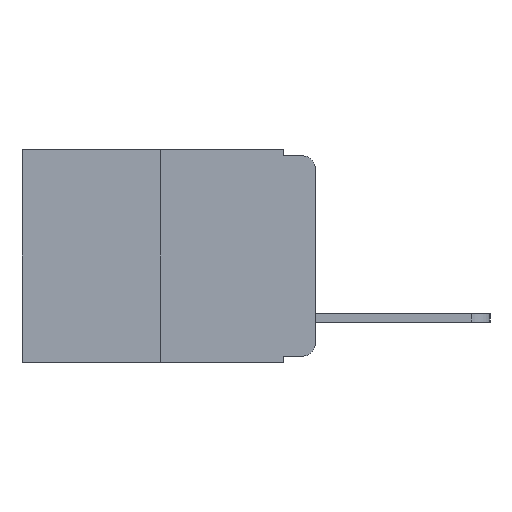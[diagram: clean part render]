
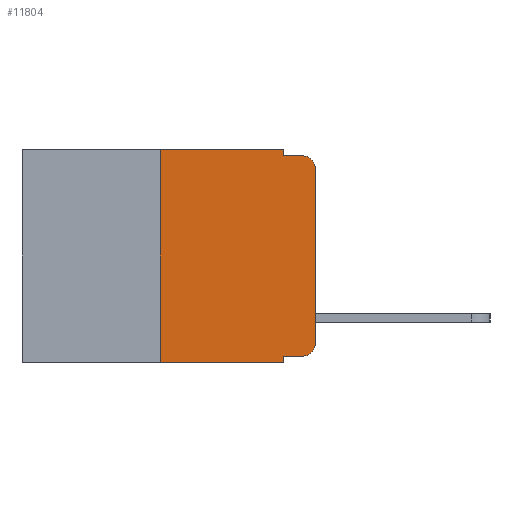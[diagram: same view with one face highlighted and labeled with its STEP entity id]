
A CAD part, left-side view. The second image highlights one B-rep face of the part: STEP entity #11804.
In plain terms, the highlighted planar face has unit normal (-1, 0, 0).
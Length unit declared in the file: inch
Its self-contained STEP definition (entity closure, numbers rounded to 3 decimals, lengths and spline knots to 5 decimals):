
#32 = CARTESIAN_POINT ( 'NONE',  ( 0., 0.051, -0.343 ) ) ;
#42 = DIRECTION ( 'NONE',  ( 0., -1., 0. ) ) ;
#110 = ORIENTED_EDGE ( 'NONE', *, *, #9940, .F. ) ;
#176 = CARTESIAN_POINT ( 'NONE',  ( 0., 0.473, -0.343 ) ) ;
#435 = DIRECTION ( 'NONE',  ( 0., -1., 0. ) ) ;
#461 = ORIENTED_EDGE ( 'NONE', *, *, #7917, .F. ) ;
#482 = CIRCLE ( 'NONE', #11625, 0.02 ) ;
#534 = VERTEX_POINT ( 'NONE', #5466 ) ;
#647 = ORIENTED_EDGE ( 'NONE', *, *, #4468, .T. ) ;
#747 = DIRECTION ( 'NONE',  ( 0., 0., -1. ) ) ;
#757 = DIRECTION ( 'NONE',  ( -1., 0., 0. ) ) ;
#991 = CARTESIAN_POINT ( 'NONE',  ( 0., 0.02, -0.313 ) ) ;
#1329 = EDGE_CURVE ( 'NONE', #7697, #7129, #11674, .T. ) ;
#1594 = LINE ( 'NONE', #12855, #9367 ) ;
#1974 = DIRECTION ( 'NONE',  ( 1., 0., 0. ) ) ;
#2759 = AXIS2_PLACEMENT_3D ( 'NONE', #12296, #1974, #9182 ) ;
#2839 = EDGE_CURVE ( 'NONE', #534, #7697, #7944, .T. ) ;
#3065 = ORIENTED_EDGE ( 'NONE', *, *, #1329, .T. ) ;
#3116 = DIRECTION ( 'NONE',  ( 0., -1., 0. ) ) ;
#3269 = DIRECTION ( 'NONE',  ( 0., 0., -1. ) ) ;
#3598 = LINE ( 'NONE', #3801, #8440 ) ;
#3801 = CARTESIAN_POINT ( 'NONE',  ( 0., 0.051, 0. ) ) ;
#3832 = LINE ( 'NONE', #6794, #9260 ) ;
#3987 = CARTESIAN_POINT ( 'NONE',  ( 0., 0.473, 0. ) ) ;
#4036 = ORIENTED_EDGE ( 'NONE', *, *, #6820, .F. ) ;
#4347 = ORIENTED_EDGE ( 'NONE', *, *, #5886, .F. ) ;
#4373 = DIRECTION ( 'NONE',  ( 0., -1., 0. ) ) ;
#4468 = EDGE_CURVE ( 'NONE', #10288, #534, #482, .T. ) ;
#5181 = EDGE_CURVE ( 'NONE', #6390, #10288, #1594, .T. ) ;
#5359 = VERTEX_POINT ( 'NONE', #7975 ) ;
#5466 = CARTESIAN_POINT ( 'NONE',  ( 0., 0., -0.313 ) ) ;
#5480 = CARTESIAN_POINT ( 'NONE',  ( 0., 0.02, -0.01 ) ) ;
#5528 = DIRECTION ( 'NONE',  ( 0., 0., -1. ) ) ;
#5850 = FACE_OUTER_BOUND ( 'NONE', #8494, .T. ) ;
#5886 = EDGE_CURVE ( 'NONE', #6390, #7399, #3598, .T. ) ;
#6109 = CARTESIAN_POINT ( 'NONE',  ( 0., 0.051, -0.333 ) ) ;
#6182 = VECTOR ( 'NONE', #42, 39.37008 ) ;
#6390 = VERTEX_POINT ( 'NONE', #6109 ) ;
#6794 = CARTESIAN_POINT ( 'NONE',  ( 0., 0.051, -0.01 ) ) ;
#6820 = EDGE_CURVE ( 'NONE', #7747, #5359, #8273, .T. ) ;
#6952 = CARTESIAN_POINT ( 'NONE',  ( 0., 0.02, -0.333 ) ) ;
#7085 = ORIENTED_EDGE ( 'NONE', *, *, #5181, .T. ) ;
#7104 = PLANE ( 'NONE',  #2759 ) ;
#7129 = VERTEX_POINT ( 'NONE', #5480 ) ;
#7214 = EDGE_CURVE ( 'NONE', #12556, #7747, #9479, .T. ) ;
#7241 = CARTESIAN_POINT ( 'NONE',  ( 0., 0.051, -0.01 ) ) ;
#7399 = VERTEX_POINT ( 'NONE', #32 ) ;
#7427 = VECTOR ( 'NONE', #11256, 39.37008 ) ;
#7446 = DIRECTION ( 'NONE',  ( 0., 0., -1. ) ) ;
#7452 = CARTESIAN_POINT ( 'NONE',  ( 0., 0., -0.03 ) ) ;
#7697 = VERTEX_POINT ( 'NONE', #7452 ) ;
#7747 = VERTEX_POINT ( 'NONE', #11300 ) ;
#7828 = EDGE_CURVE ( 'NONE', #12556, #7399, #11947, .T. ) ;
#7917 = EDGE_CURVE ( 'NONE', #5359, #10697, #10955, .T. ) ;
#7944 = LINE ( 'NONE', #8656, #13052 ) ;
#7975 = CARTESIAN_POINT ( 'NONE',  ( 0., 0.051, 0. ) ) ;
#8273 = LINE ( 'NONE', #3987, #10636 ) ;
#8440 = VECTOR ( 'NONE', #5528, 39.37008 ) ;
#8494 = EDGE_LOOP ( 'NONE', ( #13004, #3065, #110, #461, #4036, #11421, #9297, #4347, #7085, #647 ) ) ;
#8604 = DIRECTION ( 'NONE',  ( 0., 0., 1. ) ) ;
#8656 = CARTESIAN_POINT ( 'NONE',  ( 0., 0., 0. ) ) ;
#9182 = DIRECTION ( 'NONE',  ( 0., 0., -1. ) ) ;
#9260 = VECTOR ( 'NONE', #435, 39.37008 ) ;
#9297 = ORIENTED_EDGE ( 'NONE', *, *, #7828, .T. ) ;
#9367 = VECTOR ( 'NONE', #3116, 39.37008 ) ;
#9479 = LINE ( 'NONE', #11198, #7427 ) ;
#9940 = EDGE_CURVE ( 'NONE', #10697, #7129, #3832, .T. ) ;
#10011 = CARTESIAN_POINT ( 'NONE',  ( 0., 0.25, -0.343 ) ) ;
#10288 = VERTEX_POINT ( 'NONE', #6952 ) ;
#10636 = VECTOR ( 'NONE', #4373, 39.37008 ) ;
#10693 = DIRECTION ( 'NONE',  ( -1., 0., 0. ) ) ;
#10697 = VERTEX_POINT ( 'NONE', #7241 ) ;
#10825 = CARTESIAN_POINT ( 'NONE',  ( 0., 0.051, 0. ) ) ;
#10955 = LINE ( 'NONE', #10825, #13326 ) ;
#11198 = CARTESIAN_POINT ( 'NONE',  ( 0., 0.25, 0. ) ) ;
#11256 = DIRECTION ( 'NONE',  ( 0., 0., 1. ) ) ;
#11300 = CARTESIAN_POINT ( 'NONE',  ( 0., 0.25, 0. ) ) ;
#11421 = ORIENTED_EDGE ( 'NONE', *, *, #7214, .F. ) ;
#11597 = CARTESIAN_POINT ( 'NONE',  ( 0., 0.02, -0.03 ) ) ;
#11625 = AXIS2_PLACEMENT_3D ( 'NONE', #991, #757, #747 ) ;
#11674 = CIRCLE ( 'NONE', #13051, 0.02 ) ;
#11804 = ADVANCED_FACE ( 'NONE', ( #5850 ), #7104, .F. ) ;
#11947 = LINE ( 'NONE', #176, #6182 ) ;
#12296 = CARTESIAN_POINT ( 'NONE',  ( 0., 0.473, 0. ) ) ;
#12556 = VERTEX_POINT ( 'NONE', #10011 ) ;
#12855 = CARTESIAN_POINT ( 'NONE',  ( 0., 0.051, -0.333 ) ) ;
#13004 = ORIENTED_EDGE ( 'NONE', *, *, #2839, .T. ) ;
#13051 = AXIS2_PLACEMENT_3D ( 'NONE', #11597, #10693, #7446 ) ;
#13052 = VECTOR ( 'NONE', #8604, 39.37008 ) ;
#13326 = VECTOR ( 'NONE', #3269, 39.37008 ) ;
